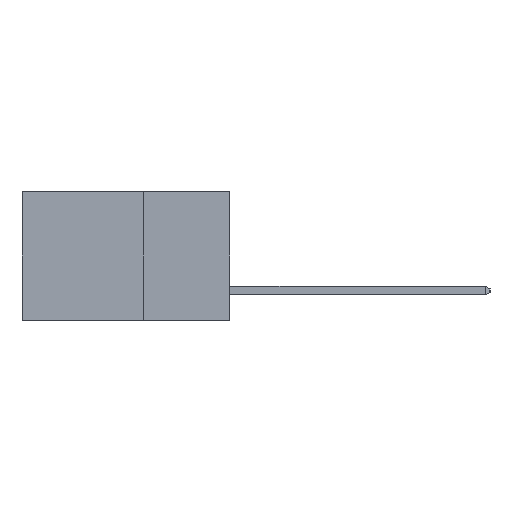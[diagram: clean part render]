
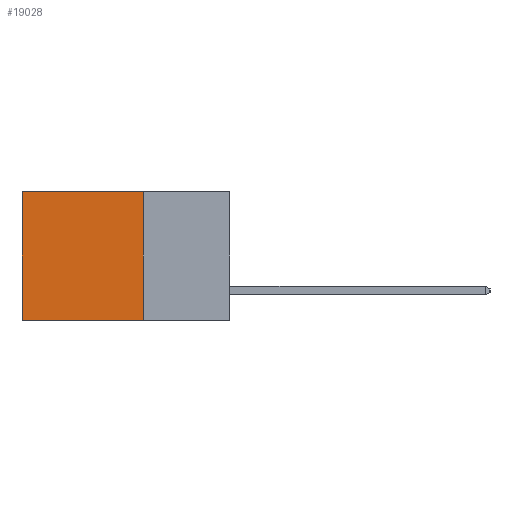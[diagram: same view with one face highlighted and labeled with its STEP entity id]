
A CAD part, left-side view. The second image highlights one B-rep face of the part: STEP entity #19028.
In plain terms, the highlighted planar face has unit normal (-1, 0, 0).
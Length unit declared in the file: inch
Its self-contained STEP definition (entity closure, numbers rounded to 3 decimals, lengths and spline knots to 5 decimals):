
#218 = LINE ( 'NONE', #12136, #4492 ) ;
#603 = CARTESIAN_POINT ( 'NONE',  ( 0.298, 0.25, 0. ) ) ;
#617 = CARTESIAN_POINT ( 'NONE',  ( 0.298, 0.25, 0. ) ) ;
#1329 = VECTOR ( 'NONE', #13703, 39.37008 ) ;
#1699 = EDGE_CURVE ( 'NONE', #10742, #7103, #9561, .T. ) ;
#2207 = ORIENTED_EDGE ( 'NONE', *, *, #1699, .T. ) ;
#2493 = CARTESIAN_POINT ( 'NONE',  ( 0.298, 0.6, -0.37 ) ) ;
#3569 = DIRECTION ( 'NONE',  ( 1., 0., 0. ) ) ;
#4492 = VECTOR ( 'NONE', #7435, 39.37008 ) ;
#5231 = VECTOR ( 'NONE', #8842, 39.37008 ) ;
#5634 = CARTESIAN_POINT ( 'NONE',  ( 0.298, 0.6, 0. ) ) ;
#5832 = EDGE_CURVE ( 'NONE', #16570, #7103, #218, .T. ) ;
#7103 = VERTEX_POINT ( 'NONE', #2493 ) ;
#7435 = DIRECTION ( 'NONE',  ( 0., 1., 0. ) ) ;
#7617 = CARTESIAN_POINT ( 'NONE',  ( 0.298, 0.25, -0.37 ) ) ;
#8842 = DIRECTION ( 'NONE',  ( 0., 0., -1. ) ) ;
#9216 = ORIENTED_EDGE ( 'NONE', *, *, #21082, .F. ) ;
#9561 = LINE ( 'NONE', #5634, #1329 ) ;
#10742 = VERTEX_POINT ( 'NONE', #12185 ) ;
#11811 = PLANE ( 'NONE',  #18404 ) ;
#12136 = CARTESIAN_POINT ( 'NONE',  ( 0.298, 0.25, -0.37 ) ) ;
#12185 = CARTESIAN_POINT ( 'NONE',  ( 0.298, 0.6, 0. ) ) ;
#13175 = VERTEX_POINT ( 'NONE', #617 ) ;
#13703 = DIRECTION ( 'NONE',  ( 0., 0., -1. ) ) ;
#14214 = DIRECTION ( 'NONE',  ( 0., 1., 0. ) ) ;
#14972 = EDGE_CURVE ( 'NONE', #13175, #10742, #19686, .T. ) ;
#15102 = DIRECTION ( 'NONE',  ( 0., 0., -1. ) ) ;
#15374 = VECTOR ( 'NONE', #14214, 39.37008 ) ;
#15626 = EDGE_LOOP ( 'NONE', ( #2207, #16305, #9216, #18672 ) ) ;
#15839 = CARTESIAN_POINT ( 'NONE',  ( 0.298, 0.25, 0. ) ) ;
#16149 = FACE_OUTER_BOUND ( 'NONE', #15626, .T. ) ;
#16305 = ORIENTED_EDGE ( 'NONE', *, *, #5832, .F. ) ;
#16570 = VERTEX_POINT ( 'NONE', #7617 ) ;
#18269 = CARTESIAN_POINT ( 'NONE',  ( 0.298, 0.25, 0. ) ) ;
#18331 = LINE ( 'NONE', #603, #5231 ) ;
#18404 = AXIS2_PLACEMENT_3D ( 'NONE', #18269, #3569, #15102 ) ;
#18672 = ORIENTED_EDGE ( 'NONE', *, *, #14972, .T. ) ;
#19028 = ADVANCED_FACE ( 'NONE', ( #16149 ), #11811, .F. ) ;
#19686 = LINE ( 'NONE', #15839, #15374 ) ;
#21082 = EDGE_CURVE ( 'NONE', #13175, #16570, #18331, .T. ) ;
